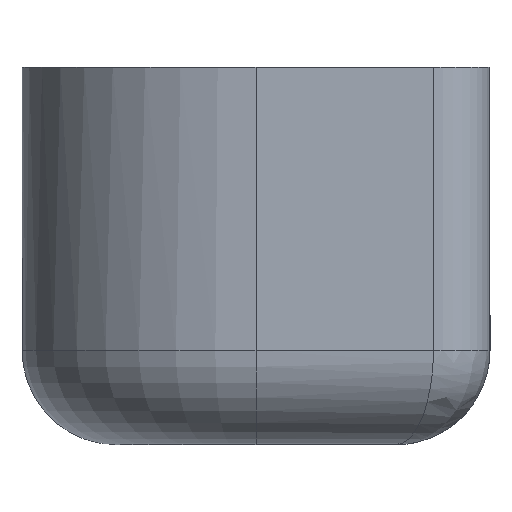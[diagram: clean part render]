
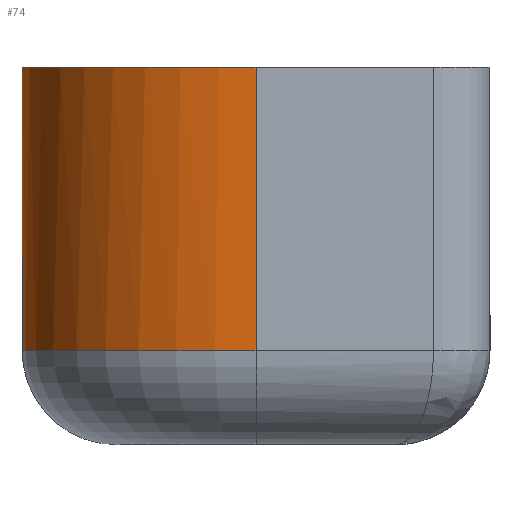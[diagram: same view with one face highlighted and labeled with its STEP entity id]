
A CAD part, left-side view. The second image highlights one B-rep face of the part: STEP entity #74.
In plain terms, the highlighted cylindrical face has radius 12.4 mm (diameter 24.8 mm), a partial arc.
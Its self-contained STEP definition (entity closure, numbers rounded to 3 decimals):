
#10 = DIRECTION ( 'NONE',  ( 0., 0., -1. ) ) ;
#30 = AXIS2_PLACEMENT_3D ( 'NONE', #975, #971, #970 ) ;
#46 = CARTESIAN_POINT ( 'NONE',  ( 107.892, 24.8, 5. ) ) ;
#74 = ADVANCED_FACE ( 'NONE', ( #267 ), #226, .T. ) ;
#113 = CARTESIAN_POINT ( 'NONE',  ( 106.991, 24.769, 20. ) ) ;
#121 = EDGE_CURVE ( 'NONE', #1131, #1165, #223, .T. ) ;
#223 = CIRCLE ( 'NONE', #30, 12.4 ) ;
#226 = CYLINDRICAL_SURFACE ( 'NONE', #746, 12.4 ) ;
#267 = FACE_OUTER_BOUND ( 'NONE', #639, .T. ) ;
#302 = CARTESIAN_POINT ( 'NONE',  ( 95.492, 12.4, 20. ) ) ;
#365 = DIRECTION ( 'NONE',  ( 0., 1., 0. ) ) ;
#370 = CARTESIAN_POINT ( 'NONE',  ( 107.53, 24.796, 19.956 ) ) ;
#381 = CARTESIAN_POINT ( 'NONE',  ( 106.81, 24.753, 20. ) ) ;
#411 = AXIS2_PLACEMENT_3D ( 'NONE', #557, #1343, #682 ) ;
#496 = CARTESIAN_POINT ( 'NONE',  ( 107.892, 24.8, 19.943 ) ) ;
#499 = VECTOR ( 'NONE', #10, 1000. ) ;
#541 = LINE ( 'NONE', #1303, #499 ) ;
#543 = VERTEX_POINT ( 'NONE', #942 ) ;
#557 = CARTESIAN_POINT ( 'NONE',  ( 107.892, 12.4, 5. ) ) ;
#561 = VERTEX_POINT ( 'NONE', #802 ) ;
#639 = EDGE_LOOP ( 'NONE', ( #715, #717, #662, #1003, #997 ) ) ;
#662 = ORIENTED_EDGE ( 'NONE', *, *, #939, .F. ) ;
#682 = DIRECTION ( 'NONE',  ( 0., 1., 0. ) ) ;
#715 = ORIENTED_EDGE ( 'NONE', *, *, #1381, .T. ) ;
#717 = ORIENTED_EDGE ( 'NONE', *, *, #1153, .T. ) ;
#721 = VERTEX_POINT ( 'NONE', #46 ) ;
#746 = AXIS2_PLACEMENT_3D ( 'NONE', #1307, #1444, #365 ) ;
#802 = CARTESIAN_POINT ( 'NONE',  ( 95.492, 12.4, 5. ) ) ;
#837 = B_SPLINE_CURVE_WITH_KNOTS ( 'NONE', 3,
 ( #381, #113, #1101, #370, #1208, #496 ),
 .UNSPECIFIED., .F., .F.,
 ( 4, 2, 4 ),
 ( 0., 0.001, 0.001 ),
 .UNSPECIFIED. ) ;
#939 = EDGE_CURVE ( 'NONE', #1165, #561, #1412, .T. ) ;
#942 = CARTESIAN_POINT ( 'NONE',  ( 107.892, 24.8, 19.943 ) ) ;
#946 = EDGE_CURVE ( 'NONE', #1131, #543, #837, .T. ) ;
#970 = DIRECTION ( 'NONE',  ( 0., 1., 0. ) ) ;
#971 = DIRECTION ( 'NONE',  ( 0., 0., 1. ) ) ;
#975 = CARTESIAN_POINT ( 'NONE',  ( 107.892, 12.4, 20. ) ) ;
#997 = ORIENTED_EDGE ( 'NONE', *, *, #946, .T. ) ;
#1000 = DIRECTION ( 'NONE',  ( 0., 0., -1. ) ) ;
#1003 = ORIENTED_EDGE ( 'NONE', *, *, #121, .F. ) ;
#1043 = CIRCLE ( 'NONE', #411, 12.4 ) ;
#1101 = CARTESIAN_POINT ( 'NONE',  ( 107.17, 24.78, 19.985 ) ) ;
#1131 = VERTEX_POINT ( 'NONE', #1409 ) ;
#1153 = EDGE_CURVE ( 'NONE', #721, #561, #1043, .T. ) ;
#1165 = VERTEX_POINT ( 'NONE', #302 ) ;
#1208 = CARTESIAN_POINT ( 'NONE',  ( 107.711, 24.8, 19.943 ) ) ;
#1252 = CARTESIAN_POINT ( 'NONE',  ( 95.492, 12.4, 214.388 ) ) ;
#1303 = CARTESIAN_POINT ( 'NONE',  ( 107.892, 24.8, 214.388 ) ) ;
#1307 = CARTESIAN_POINT ( 'NONE',  ( 107.892, 12.4, 214.388 ) ) ;
#1343 = DIRECTION ( 'NONE',  ( 0., 0., 1. ) ) ;
#1373 = VECTOR ( 'NONE', #1000, 1000. ) ;
#1381 = EDGE_CURVE ( 'NONE', #543, #721, #541, .T. ) ;
#1409 = CARTESIAN_POINT ( 'NONE',  ( 106.81, 24.753, 20. ) ) ;
#1412 = LINE ( 'NONE', #1252, #1373 ) ;
#1444 = DIRECTION ( 'NONE',  ( 0., 0., -1. ) ) ;
